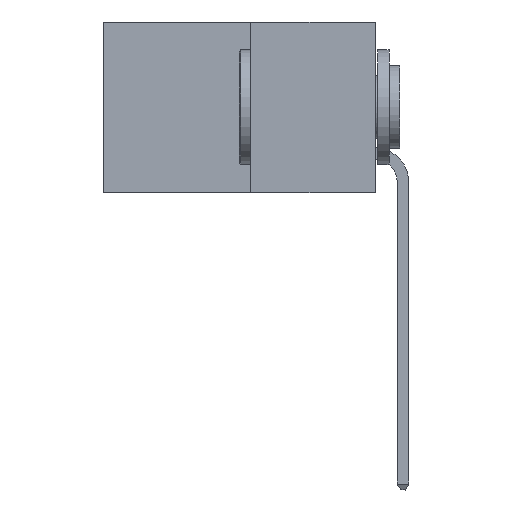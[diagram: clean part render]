
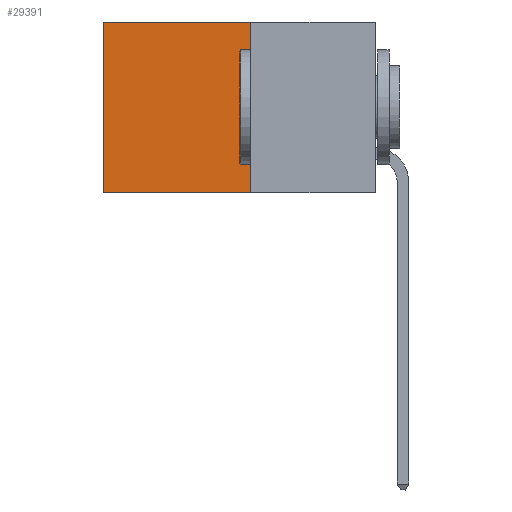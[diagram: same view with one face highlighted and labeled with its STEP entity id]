
A CAD part, left-side view. The second image highlights one B-rep face of the part: STEP entity #29391.
In plain terms, the highlighted planar face has unit normal (-1, 0, 0).
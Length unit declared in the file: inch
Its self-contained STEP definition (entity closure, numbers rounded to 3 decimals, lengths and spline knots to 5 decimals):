
#61 = LINE ( 'NONE', #30605, #12616 ) ;
#670 = FACE_OUTER_BOUND ( 'NONE', #29856, .T. ) ;
#1208 = LINE ( 'NONE', #19448, #25615 ) ;
#1755 = CARTESIAN_POINT ( 'NONE',  ( 0.277, 0.27, 0. ) ) ;
#2714 = CARTESIAN_POINT ( 'NONE',  ( 0.277, 0.27, 0. ) ) ;
#4604 = AXIS2_PLACEMENT_3D ( 'NONE', #19295, #21847, #6832 ) ;
#4911 = VECTOR ( 'NONE', #19315, 39.37008 ) ;
#5572 = DIRECTION ( 'NONE',  ( 0., 0., -1. ) ) ;
#5937 = EDGE_CURVE ( 'NONE', #6495, #30664, #18823, .T. ) ;
#6495 = VERTEX_POINT ( 'NONE', #25351 ) ;
#6832 = DIRECTION ( 'NONE',  ( 0., 0., -1. ) ) ;
#8104 = CARTESIAN_POINT ( 'NONE',  ( 0.277, 0.27, -0.37 ) ) ;
#8583 = EDGE_CURVE ( 'NONE', #12696, #21058, #24981, .T. ) ;
#9588 = EDGE_CURVE ( 'NONE', #21058, #30664, #61, .T. ) ;
#11323 = EDGE_CURVE ( 'NONE', #12696, #6495, #1208, .T. ) ;
#12616 = VECTOR ( 'NONE', #5572, 39.37008 ) ;
#12696 = VERTEX_POINT ( 'NONE', #2714 ) ;
#14638 = CARTESIAN_POINT ( 'NONE',  ( 0.277, 0.59, -0.37 ) ) ;
#15148 = ORIENTED_EDGE ( 'NONE', *, *, #9588, .T. ) ;
#16088 = ORIENTED_EDGE ( 'NONE', *, *, #11323, .F. ) ;
#16738 = PLANE ( 'NONE',  #4604 ) ;
#17679 = ORIENTED_EDGE ( 'NONE', *, *, #8583, .T. ) ;
#18019 = VECTOR ( 'NONE', #20619, 39.37008 ) ;
#18823 = LINE ( 'NONE', #8104, #18019 ) ;
#19295 = CARTESIAN_POINT ( 'NONE',  ( 0.277, 0.27, -0.37 ) ) ;
#19315 = DIRECTION ( 'NONE',  ( 0., 1., 0. ) ) ;
#19448 = CARTESIAN_POINT ( 'NONE',  ( 0.277, 0.27, -0.37 ) ) ;
#20619 = DIRECTION ( 'NONE',  ( 0., 1., 0. ) ) ;
#21058 = VERTEX_POINT ( 'NONE', #30432 ) ;
#21847 = DIRECTION ( 'NONE',  ( 1., 0., 0. ) ) ;
#22005 = DIRECTION ( 'NONE',  ( 0., 0., -1. ) ) ;
#24603 = ORIENTED_EDGE ( 'NONE', *, *, #5937, .F. ) ;
#24981 = LINE ( 'NONE', #1755, #4911 ) ;
#25351 = CARTESIAN_POINT ( 'NONE',  ( 0.277, 0.27, -0.37 ) ) ;
#25615 = VECTOR ( 'NONE', #22005, 39.37008 ) ;
#29391 = ADVANCED_FACE ( 'NONE', ( #670 ), #16738, .F. ) ;
#29856 = EDGE_LOOP ( 'NONE', ( #15148, #24603, #16088, #17679 ) ) ;
#30432 = CARTESIAN_POINT ( 'NONE',  ( 0.277, 0.59, 0. ) ) ;
#30605 = CARTESIAN_POINT ( 'NONE',  ( 0.277, 0.59, -0.37 ) ) ;
#30664 = VERTEX_POINT ( 'NONE', #14638 ) ;
